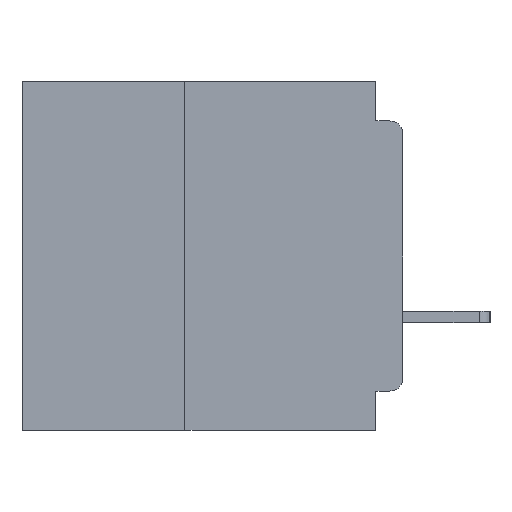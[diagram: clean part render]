
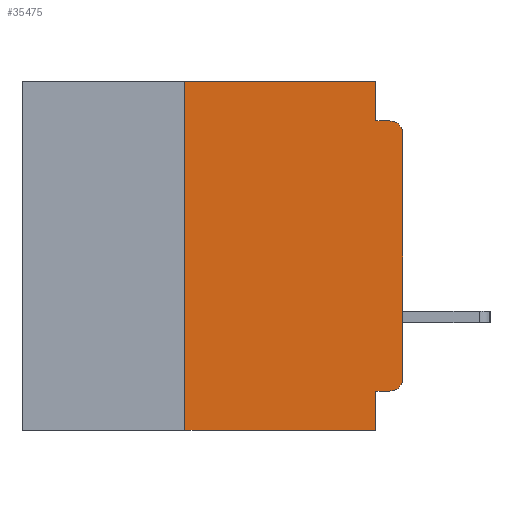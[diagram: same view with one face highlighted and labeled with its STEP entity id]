
A CAD part, left-side view. The second image highlights one B-rep face of the part: STEP entity #35475.
In plain terms, the highlighted planar face has unit normal (-1, 0, 0).
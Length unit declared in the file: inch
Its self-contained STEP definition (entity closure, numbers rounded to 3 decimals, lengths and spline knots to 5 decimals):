
#1164 = LINE ( 'NONE', #25329, #34718 ) ;
#1448 = LINE ( 'NONE', #28508, #26233 ) ;
#1854 = PLANE ( 'NONE',  #13692 ) ;
#2006 = DIRECTION ( 'NONE',  ( 0., 0., -1. ) ) ;
#4194 = VERTEX_POINT ( 'NONE', #18568 ) ;
#4977 = VERTEX_POINT ( 'NONE', #5731 ) ;
#5045 = LINE ( 'NONE', #28375, #22945 ) ;
#5529 = VERTEX_POINT ( 'NONE', #9365 ) ;
#5731 = CARTESIAN_POINT ( 'NONE',  ( 0., 0.25, 0. ) ) ;
#6800 = VECTOR ( 'NONE', #12794, 39.37008 ) ;
#7227 = VERTEX_POINT ( 'NONE', #23185 ) ;
#8274 = VECTOR ( 'NONE', #40465, 39.37008 ) ;
#8358 = DIRECTION ( 'NONE',  ( 0., 1., 0. ) ) ;
#8620 = DIRECTION ( 'NONE',  ( 0., 0., 1. ) ) ;
#9365 = CARTESIAN_POINT ( 'NONE',  ( 0., 0., -0.06 ) ) ;
#9406 = EDGE_CURVE ( 'NONE', #7227, #29704, #1448, .T. ) ;
#9565 = CARTESIAN_POINT ( 'NONE',  ( 0., 0.031, 0. ) ) ;
#11212 = EDGE_CURVE ( 'NONE', #37336, #7227, #5045, .T. ) ;
#11842 = DIRECTION ( 'NONE',  ( -1., 0., 0. ) ) ;
#12011 = DIRECTION ( 'NONE',  ( 0., -1., 0. ) ) ;
#12136 = AXIS2_PLACEMENT_3D ( 'NONE', #33787, #13869, #37097 ) ;
#12285 = VECTOR ( 'NONE', #14244, 39.37008 ) ;
#12794 = DIRECTION ( 'NONE',  ( 0., 0., -1. ) ) ;
#12800 = VECTOR ( 'NONE', #8620, 39.37008 ) ;
#12892 = EDGE_CURVE ( 'NONE', #37336, #42591, #42410, .T. ) ;
#13400 = VERTEX_POINT ( 'NONE', #23074 ) ;
#13692 = AXIS2_PLACEMENT_3D ( 'NONE', #42011, #22211, #2006 ) ;
#13869 = DIRECTION ( 'NONE',  ( -1., 0., 0. ) ) ;
#14244 = DIRECTION ( 'NONE',  ( 0., -1., 0. ) ) ;
#16235 = CARTESIAN_POINT ( 'NONE',  ( 0., 0.015, -0.355 ) ) ;
#16382 = EDGE_CURVE ( 'NONE', #31484, #29704, #38817, .T. ) ;
#16829 = CARTESIAN_POINT ( 'NONE',  ( 0., 0., -0.34 ) ) ;
#17161 = DIRECTION ( 'NONE',  ( 0., -1., 0. ) ) ;
#17474 = ORIENTED_EDGE ( 'NONE', *, *, #24457, .F. ) ;
#18568 = CARTESIAN_POINT ( 'NONE',  ( 0., 0.031, -0.045 ) ) ;
#18765 = ORIENTED_EDGE ( 'NONE', *, *, #34290, .F. ) ;
#20177 = LINE ( 'NONE', #34133, #12285 ) ;
#20178 = EDGE_LOOP ( 'NONE', ( #27750, #27554, #17474, #18765, #23062, #20947, #22226, #34914, #22163, #21377 ) ) ;
#20947 = ORIENTED_EDGE ( 'NONE', *, *, #24682, .F. ) ;
#21222 = VECTOR ( 'NONE', #17161, 39.37008 ) ;
#21377 = ORIENTED_EDGE ( 'NONE', *, *, #12892, .T. ) ;
#21712 = LINE ( 'NONE', #25314, #12800 ) ;
#22163 = ORIENTED_EDGE ( 'NONE', *, *, #11212, .F. ) ;
#22211 = DIRECTION ( 'NONE',  ( 1., 0., 0. ) ) ;
#22226 = ORIENTED_EDGE ( 'NONE', *, *, #16382, .T. ) ;
#22945 = VECTOR ( 'NONE', #8358, 39.37008 ) ;
#23062 = ORIENTED_EDGE ( 'NONE', *, *, #36569, .F. ) ;
#23074 = CARTESIAN_POINT ( 'NONE',  ( 0., 0.031, 0. ) ) ;
#23185 = CARTESIAN_POINT ( 'NONE',  ( 0., 0.031, -0.355 ) ) ;
#23235 = CARTESIAN_POINT ( 'NONE',  ( 0., 0.015, -0.045 ) ) ;
#24457 = EDGE_CURVE ( 'NONE', #4194, #38882, #20177, .T. ) ;
#24682 = EDGE_CURVE ( 'NONE', #31484, #4977, #21712, .T. ) ;
#25314 = CARTESIAN_POINT ( 'NONE',  ( 0., 0.25, -0.4 ) ) ;
#25329 = CARTESIAN_POINT ( 'NONE',  ( 0., 0.437, 0. ) ) ;
#26233 = VECTOR ( 'NONE', #38437, 39.37008 ) ;
#26488 = EDGE_CURVE ( 'NONE', #5529, #38882, #27262, .T. ) ;
#26597 = FACE_OUTER_BOUND ( 'NONE', #20178, .T. ) ;
#27250 = CARTESIAN_POINT ( 'NONE',  ( 0., 0.25, -0.4 ) ) ;
#27262 = CIRCLE ( 'NONE', #28503, 0.015 ) ;
#27554 = ORIENTED_EDGE ( 'NONE', *, *, #26488, .T. ) ;
#27750 = ORIENTED_EDGE ( 'NONE', *, *, #42079, .T. ) ;
#28375 = CARTESIAN_POINT ( 'NONE',  ( 0., 0., -0.355 ) ) ;
#28503 = AXIS2_PLACEMENT_3D ( 'NONE', #31800, #11842, #35114 ) ;
#28508 = CARTESIAN_POINT ( 'NONE',  ( 0., 0.031, -0.4 ) ) ;
#29704 = VERTEX_POINT ( 'NONE', #33882 ) ;
#31484 = VERTEX_POINT ( 'NONE', #27250 ) ;
#31800 = CARTESIAN_POINT ( 'NONE',  ( 0., 0.015, -0.06 ) ) ;
#33406 = LINE ( 'NONE', #9565, #6800 ) ;
#33705 = CARTESIAN_POINT ( 'NONE',  ( 0., 0.437, -0.4 ) ) ;
#33787 = CARTESIAN_POINT ( 'NONE',  ( 0., 0.015, -0.34 ) ) ;
#33882 = CARTESIAN_POINT ( 'NONE',  ( 0., 0.031, -0.4 ) ) ;
#34133 = CARTESIAN_POINT ( 'NONE',  ( 0., 0., -0.045 ) ) ;
#34290 = EDGE_CURVE ( 'NONE', #13400, #4194, #33406, .T. ) ;
#34718 = VECTOR ( 'NONE', #12011, 39.37008 ) ;
#34844 = LINE ( 'NONE', #37152, #8274 ) ;
#34914 = ORIENTED_EDGE ( 'NONE', *, *, #9406, .F. ) ;
#35114 = DIRECTION ( 'NONE',  ( 0., 0., -1. ) ) ;
#35475 = ADVANCED_FACE ( 'NONE', ( #26597 ), #1854, .F. ) ;
#36569 = EDGE_CURVE ( 'NONE', #4977, #13400, #1164, .T. ) ;
#37097 = DIRECTION ( 'NONE',  ( 0., 0., -1. ) ) ;
#37152 = CARTESIAN_POINT ( 'NONE',  ( 0., 0., 0. ) ) ;
#37336 = VERTEX_POINT ( 'NONE', #16235 ) ;
#38437 = DIRECTION ( 'NONE',  ( 0., 0., -1. ) ) ;
#38817 = LINE ( 'NONE', #33705, #21222 ) ;
#38882 = VERTEX_POINT ( 'NONE', #23235 ) ;
#40465 = DIRECTION ( 'NONE',  ( 0., 0., 1. ) ) ;
#42011 = CARTESIAN_POINT ( 'NONE',  ( 0., 0.437, 0. ) ) ;
#42079 = EDGE_CURVE ( 'NONE', #42591, #5529, #34844, .T. ) ;
#42410 = CIRCLE ( 'NONE', #12136, 0.015 ) ;
#42591 = VERTEX_POINT ( 'NONE', #16829 ) ;
